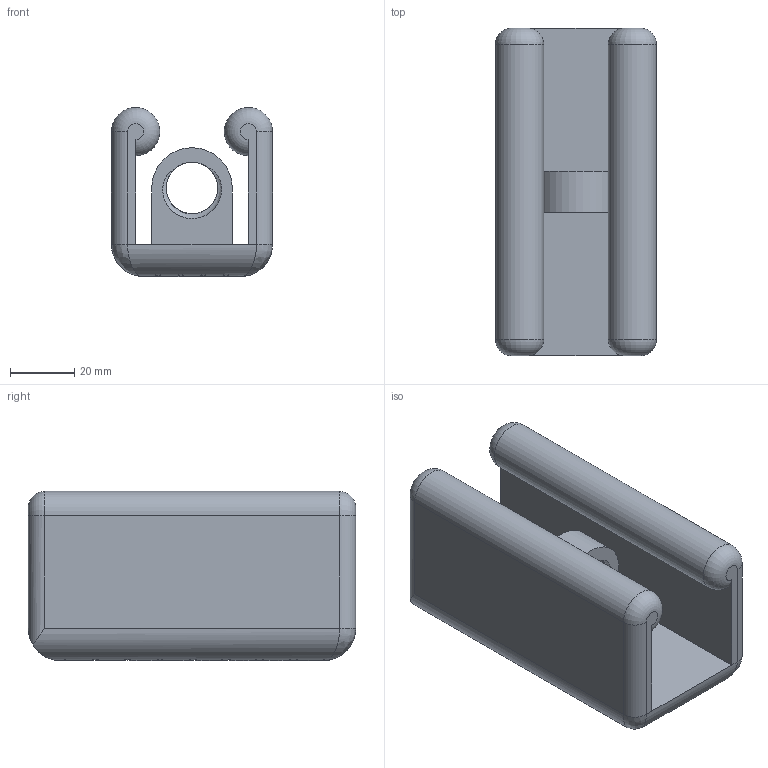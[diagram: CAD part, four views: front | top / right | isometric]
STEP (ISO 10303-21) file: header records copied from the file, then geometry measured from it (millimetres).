
FILE_DESCRIPTION (( 'STEP AP214' ), '1' );
FILE_NAME ('Trellais_Rear_Plate.step', '2016-04-19T10:44:38', ( 'WarFairy' ), ( '' ), 'SwSTEP 2.0', 'SolidWorks 2015', '' );
FILE_SCHEMA (( 'AUTOMOTIVE_DESIGN' ));
Length unit declared in the file: millimetre
Products named in the file (1): Trellais_Rear_Plate
Bounding box: 50 x 101.6 x 52.5 mm (x, y, z)
Volume: 128446.2 mm3; surface area: 34382.1 mm2
Topology: 1 solids, 1 shells, 2962 faces, 5920 edges, 2958 vertices
Faces by surface type: cone 2418, plane 432, cylinder 101, bspline 7, torus 4
Entity records: 80776 total; most frequent: CARTESIAN_POINT 24976, ORIENTED_EDGE 11834, DIRECTION 11488, EDGE_CURVE 5917, AXIS2_PLACEMENT_3D 5679, B_SPLINE_CURVE_WITH_KNOTS 3056, EDGE_LOOP 2965, ADVANCED_FACE 2962
